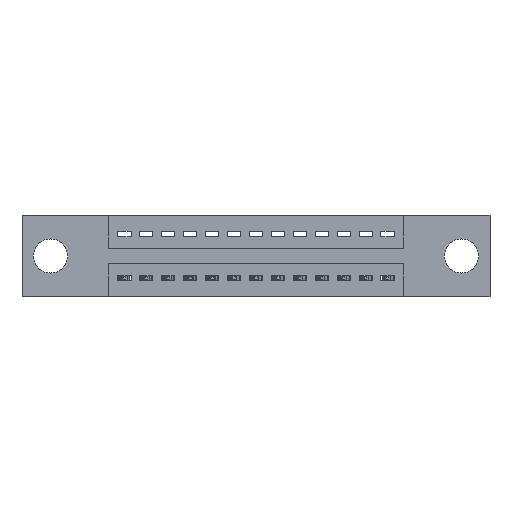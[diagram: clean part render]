
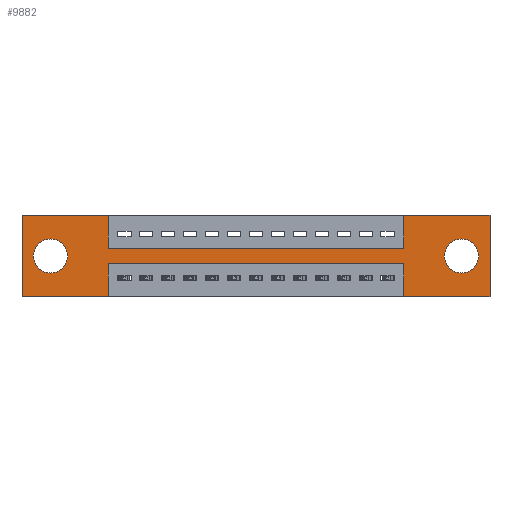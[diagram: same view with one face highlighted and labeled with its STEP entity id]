
A CAD part, front view. The second image highlights one B-rep face of the part: STEP entity #9882.
In plain terms, the highlighted planar face has unit normal (0, -1, 0).
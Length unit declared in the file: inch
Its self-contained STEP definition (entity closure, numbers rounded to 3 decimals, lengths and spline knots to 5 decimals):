
#32 = EDGE_CURVE ( 'NONE', #3454, #3719, #2031, .T. ) ;
#58 = VECTOR ( 'NONE', #12045, 39.37008 ) ;
#143 = VERTEX_POINT ( 'NONE', #7067 ) ;
#251 = VERTEX_POINT ( 'NONE', #1106 ) ;
#373 = EDGE_CURVE ( 'NONE', #11294, #251, #3180, .T. ) ;
#689 = ORIENTED_EDGE ( 'NONE', *, *, #10907, .T. ) ;
#942 = VERTEX_POINT ( 'NONE', #3061 ) ;
#966 = CARTESIAN_POINT ( 'NONE',  ( 0., 0., 0. ) ) ;
#1106 = CARTESIAN_POINT ( 'NONE',  ( 2.135, 0., 0. ) ) ;
#1173 = CARTESIAN_POINT ( 'NONE',  ( 0.3925, 0., -0.37 ) ) ;
#1224 = LINE ( 'NONE', #10007, #58 ) ;
#1230 = ORIENTED_EDGE ( 'NONE', *, *, #7532, .F. ) ;
#1293 = CARTESIAN_POINT ( 'NONE',  ( 0.3925, 0., 0. ) ) ;
#1326 = VERTEX_POINT ( 'NONE', #5556 ) ;
#1365 = VERTEX_POINT ( 'NONE', #6508 ) ;
#1479 = VERTEX_POINT ( 'NONE', #11125 ) ;
#1516 = CARTESIAN_POINT ( 'NONE',  ( 2.005, 0., -0.263 ) ) ;
#1696 = EDGE_LOOP ( 'NONE', ( #689, #4367 ) ) ;
#1842 = VERTEX_POINT ( 'NONE', #3892 ) ;
#1844 = EDGE_CURVE ( 'NONE', #12276, #12826, #6912, .T. ) ;
#1934 = VECTOR ( 'NONE', #1947, 39.37008 ) ;
#1947 = DIRECTION ( 'NONE',  ( -1., 0., 0. ) ) ;
#2031 = LINE ( 'NONE', #11075, #7330 ) ;
#2492 = ORIENTED_EDGE ( 'NONE', *, *, #373, .F. ) ;
#2785 = ORIENTED_EDGE ( 'NONE', *, *, #9589, .F. ) ;
#2919 = EDGE_CURVE ( 'NONE', #6062, #10909, #4741, .T. ) ;
#2964 = DIRECTION ( 'NONE',  ( 0., 1., 0. ) ) ;
#3061 = CARTESIAN_POINT ( 'NONE',  ( 0.13, 0., -0.263 ) ) ;
#3180 = LINE ( 'NONE', #5908, #3841 ) ;
#3309 = EDGE_CURVE ( 'NONE', #12571, #11294, #10048, .T. ) ;
#3338 = DIRECTION ( 'NONE',  ( 0., 0., -1. ) ) ;
#3454 = VERTEX_POINT ( 'NONE', #966 ) ;
#3719 = VERTEX_POINT ( 'NONE', #12350 ) ;
#3783 = AXIS2_PLACEMENT_3D ( 'NONE', #11159, #4831, #9072 ) ;
#3841 = VECTOR ( 'NONE', #11195, 39.37008 ) ;
#3848 = VERTEX_POINT ( 'NONE', #13677 ) ;
#3892 = CARTESIAN_POINT ( 'NONE',  ( 2.135, 0., -0.37 ) ) ;
#3986 = CARTESIAN_POINT ( 'NONE',  ( 1.7425, 0., -0.15 ) ) ;
#4075 = ORIENTED_EDGE ( 'NONE', *, *, #7323, .F. ) ;
#4152 = AXIS2_PLACEMENT_3D ( 'NONE', #6048, #2964, #5045 ) ;
#4213 = CARTESIAN_POINT ( 'NONE',  ( 0.13, 0., -0.185 ) ) ;
#4367 = ORIENTED_EDGE ( 'NONE', *, *, #6146, .T. ) ;
#4652 = CARTESIAN_POINT ( 'NONE',  ( 0., 0., -0.37 ) ) ;
#4681 = ORIENTED_EDGE ( 'NONE', *, *, #2919, .F. ) ;
#4740 = DIRECTION ( 'NONE',  ( 1., 0., 0. ) ) ;
#4741 = LINE ( 'NONE', #10419, #1934 ) ;
#4831 = DIRECTION ( 'NONE',  ( 0., 1., 0. ) ) ;
#5022 = ORIENTED_EDGE ( 'NONE', *, *, #11964, .T. ) ;
#5029 = DIRECTION ( 'NONE',  ( 1., 0., 0. ) ) ;
#5045 = DIRECTION ( 'NONE',  ( 0., 0., -1. ) ) ;
#5071 = CARTESIAN_POINT ( 'NONE',  ( 1.7425, 0., 0. ) ) ;
#5243 = CARTESIAN_POINT ( 'NONE',  ( 0., 0., -0.37 ) ) ;
#5273 = CARTESIAN_POINT ( 'NONE',  ( 0., 0., -0.37 ) ) ;
#5500 = LINE ( 'NONE', #6028, #9812 ) ;
#5556 = CARTESIAN_POINT ( 'NONE',  ( 1.7425, 0., -0.37 ) ) ;
#5750 = ORIENTED_EDGE ( 'NONE', *, *, #5910, .F. ) ;
#5756 = DIRECTION ( 'NONE',  ( -1., 0., 0. ) ) ;
#5852 = ORIENTED_EDGE ( 'NONE', *, *, #32, .F. ) ;
#5908 = CARTESIAN_POINT ( 'NONE',  ( 0., 0., 0. ) ) ;
#5910 = EDGE_CURVE ( 'NONE', #1365, #143, #8857, .T. ) ;
#5974 = ORIENTED_EDGE ( 'NONE', *, *, #10464, .F. ) ;
#6028 = CARTESIAN_POINT ( 'NONE',  ( 0.3925, 0., -0.15 ) ) ;
#6048 = CARTESIAN_POINT ( 'NONE',  ( 2.005, 0., -0.185 ) ) ;
#6062 = VERTEX_POINT ( 'NONE', #9170 ) ;
#6140 = CARTESIAN_POINT ( 'NONE',  ( 2.005, 0., -0.185 ) ) ;
#6146 = EDGE_CURVE ( 'NONE', #942, #1479, #8548, .T. ) ;
#6471 = AXIS2_PLACEMENT_3D ( 'NONE', #5243, #13589, #12574 ) ;
#6485 = LINE ( 'NONE', #6670, #8484 ) ;
#6508 = CARTESIAN_POINT ( 'NONE',  ( 1.7425, 0., -0.22 ) ) ;
#6670 = CARTESIAN_POINT ( 'NONE',  ( 2.135, 0., 0. ) ) ;
#6912 = CIRCLE ( 'NONE', #4152, 0.078 ) ;
#7017 = VECTOR ( 'NONE', #5756, 39.37008 ) ;
#7067 = CARTESIAN_POINT ( 'NONE',  ( 0.3925, 0., -0.22 ) ) ;
#7139 = FACE_BOUND ( 'NONE', #11258, .T. ) ;
#7227 = DIRECTION ( 'NONE',  ( 0., 0., -1. ) ) ;
#7293 = AXIS2_PLACEMENT_3D ( 'NONE', #6140, #13569, #7227 ) ;
#7323 = EDGE_CURVE ( 'NONE', #1842, #1326, #8982, .T. ) ;
#7330 = VECTOR ( 'NONE', #4740, 39.37008 ) ;
#7532 = EDGE_CURVE ( 'NONE', #3848, #12571, #5500, .T. ) ;
#7647 = VECTOR ( 'NONE', #10811, 39.37008 ) ;
#7799 = DIRECTION ( 'NONE',  ( -1., 0., 0. ) ) ;
#7901 = CARTESIAN_POINT ( 'NONE',  ( 0.3925, 0., -0.22 ) ) ;
#8005 = CIRCLE ( 'NONE', #10657, 0.078 ) ;
#8040 = ORIENTED_EDGE ( 'NONE', *, *, #8950, .F. ) ;
#8231 = DIRECTION ( 'NONE',  ( 0., 0., 1. ) ) ;
#8442 = PLANE ( 'NONE',  #6471 ) ;
#8484 = VECTOR ( 'NONE', #11966, 39.37008 ) ;
#8548 = CIRCLE ( 'NONE', #3783, 0.078 ) ;
#8639 = ORIENTED_EDGE ( 'NONE', *, *, #11669, .F. ) ;
#8857 = LINE ( 'NONE', #7901, #12687 ) ;
#8950 = EDGE_CURVE ( 'NONE', #251, #1842, #6485, .T. ) ;
#8982 = LINE ( 'NONE', #4652, #7017 ) ;
#9072 = DIRECTION ( 'NONE',  ( 0., 0., 1. ) ) ;
#9170 = CARTESIAN_POINT ( 'NONE',  ( 0.3925, 0., -0.37 ) ) ;
#9233 = CARTESIAN_POINT ( 'NONE',  ( 1.7425, 0., 0. ) ) ;
#9446 = CARTESIAN_POINT ( 'NONE',  ( 0., 0., 0. ) ) ;
#9589 = EDGE_CURVE ( 'NONE', #3719, #3848, #9633, .T. ) ;
#9604 = ORIENTED_EDGE ( 'NONE', *, *, #3309, .F. ) ;
#9627 = EDGE_LOOP ( 'NONE', ( #5974, #5750, #8639, #4075, #8040, #2492, #9604, #1230, #2785, #5852, #13714, #4681 ) ) ;
#9633 = LINE ( 'NONE', #1293, #7647 ) ;
#9812 = VECTOR ( 'NONE', #5029, 39.37008 ) ;
#9882 = ADVANCED_FACE ( 'NONE', ( #7139, #11756, #13244 ), #8442, .T. ) ;
#9950 = CARTESIAN_POINT ( 'NONE',  ( 2.005, 0., -0.107 ) ) ;
#9964 = CIRCLE ( 'NONE', #7293, 0.078 ) ;
#10007 = CARTESIAN_POINT ( 'NONE',  ( 1.7425, 0., -0.37 ) ) ;
#10048 = LINE ( 'NONE', #5071, #11862 ) ;
#10306 = VECTOR ( 'NONE', #11472, 39.37008 ) ;
#10419 = CARTESIAN_POINT ( 'NONE',  ( 0., 0., -0.37 ) ) ;
#10464 = EDGE_CURVE ( 'NONE', #143, #6062, #11579, .T. ) ;
#10657 = AXIS2_PLACEMENT_3D ( 'NONE', #4213, #11522, #11613 ) ;
#10811 = DIRECTION ( 'NONE',  ( 0., 0., -1. ) ) ;
#10907 = EDGE_CURVE ( 'NONE', #1479, #942, #8005, .T. ) ;
#10909 = VERTEX_POINT ( 'NONE', #5273 ) ;
#11075 = CARTESIAN_POINT ( 'NONE',  ( 0., 0., 0. ) ) ;
#11107 = LINE ( 'NONE', #9446, #10306 ) ;
#11125 = CARTESIAN_POINT ( 'NONE',  ( 0.13, 0., -0.107 ) ) ;
#11159 = CARTESIAN_POINT ( 'NONE',  ( 0.13, 0., -0.185 ) ) ;
#11195 = DIRECTION ( 'NONE',  ( 1., 0., 0. ) ) ;
#11258 = EDGE_LOOP ( 'NONE', ( #5022, #11953 ) ) ;
#11294 = VERTEX_POINT ( 'NONE', #9233 ) ;
#11472 = DIRECTION ( 'NONE',  ( 0., 0., 1. ) ) ;
#11522 = DIRECTION ( 'NONE',  ( 0., 1., 0. ) ) ;
#11579 = LINE ( 'NONE', #1173, #12731 ) ;
#11613 = DIRECTION ( 'NONE',  ( 0., 0., 1. ) ) ;
#11669 = EDGE_CURVE ( 'NONE', #1326, #1365, #1224, .T. ) ;
#11756 = FACE_BOUND ( 'NONE', #1696, .T. ) ;
#11862 = VECTOR ( 'NONE', #8231, 39.37008 ) ;
#11886 = EDGE_CURVE ( 'NONE', #10909, #3454, #11107, .T. ) ;
#11953 = ORIENTED_EDGE ( 'NONE', *, *, #1844, .T. ) ;
#11964 = EDGE_CURVE ( 'NONE', #12826, #12276, #9964, .T. ) ;
#11966 = DIRECTION ( 'NONE',  ( 0., 0., -1. ) ) ;
#12045 = DIRECTION ( 'NONE',  ( 0., 0., 1. ) ) ;
#12276 = VERTEX_POINT ( 'NONE', #1516 ) ;
#12350 = CARTESIAN_POINT ( 'NONE',  ( 0.3925, 0., 0. ) ) ;
#12571 = VERTEX_POINT ( 'NONE', #3986 ) ;
#12574 = DIRECTION ( 'NONE',  ( 0., 0., -1. ) ) ;
#12687 = VECTOR ( 'NONE', #7799, 39.37008 ) ;
#12731 = VECTOR ( 'NONE', #3338, 39.37008 ) ;
#12826 = VERTEX_POINT ( 'NONE', #9950 ) ;
#13244 = FACE_OUTER_BOUND ( 'NONE', #9627, .T. ) ;
#13569 = DIRECTION ( 'NONE',  ( 0., 1., 0. ) ) ;
#13589 = DIRECTION ( 'NONE',  ( 0., -1., 0. ) ) ;
#13677 = CARTESIAN_POINT ( 'NONE',  ( 0.3925, 0., -0.15 ) ) ;
#13714 = ORIENTED_EDGE ( 'NONE', *, *, #11886, .F. ) ;
